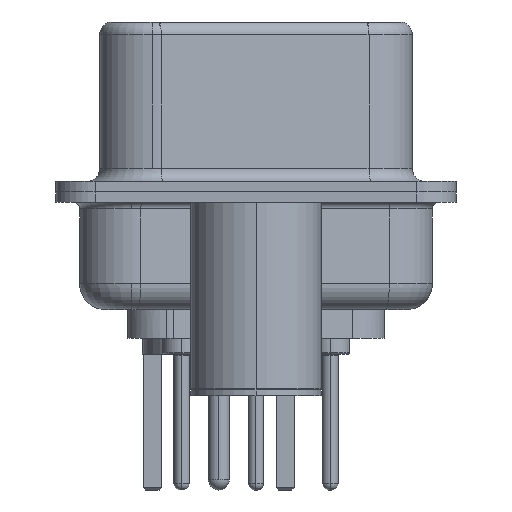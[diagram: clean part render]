
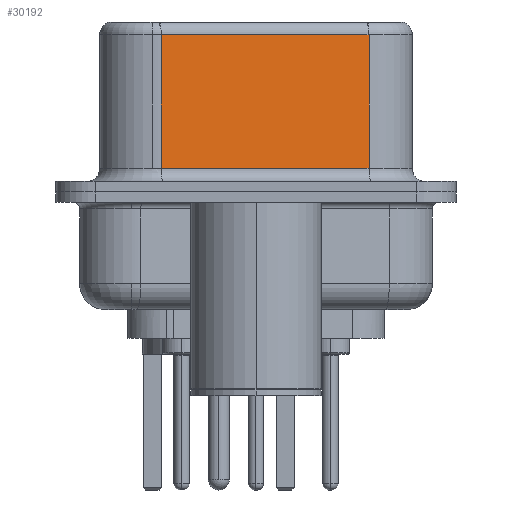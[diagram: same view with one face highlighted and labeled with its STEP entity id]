
A CAD part, left-side view. The second image highlights one B-rep face of the part: STEP entity #30192.
In plain terms, the highlighted planar face has unit normal (-0.985, -0.174, 0).
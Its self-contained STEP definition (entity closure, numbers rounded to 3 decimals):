
#232 = ORIENTED_EDGE ( 'NONE', *, *, #10060, .T. ) ;
#442 = CARTESIAN_POINT ( 'NONE',  ( 3.73, 3.628, 6.52 ) ) ;
#1006 = DIRECTION ( 'NONE',  ( 0., 0., -1. ) ) ;
#1136 = EDGE_CURVE ( 'NONE', #17221, #1732, #16563, .T. ) ;
#1732 = VERTEX_POINT ( 'NONE', #21829 ) ;
#3690 = AXIS2_PLACEMENT_3D ( 'NONE', #26724, #10558, #29506 ) ;
#3883 = VECTOR ( 'NONE', #21777, 1000. ) ;
#4448 = CARTESIAN_POINT ( 'NONE',  ( 3.73, 3.628, 0.9 ) ) ;
#5044 = PLANE ( 'NONE',  #3690 ) ;
#6447 = CARTESIAN_POINT ( 'NONE',  ( 5.132, -4.322, 0.9 ) ) ;
#8502 = VECTOR ( 'NONE', #10737, 1000. ) ;
#9507 = VECTOR ( 'NONE', #1006, 1000. ) ;
#9633 = EDGE_CURVE ( 'NONE', #17221, #12766, #16717, .T. ) ;
#10060 = EDGE_CURVE ( 'NONE', #15599, #12766, #18360, .T. ) ;
#10193 = LINE ( 'NONE', #442, #23711 ) ;
#10558 = DIRECTION ( 'NONE',  ( 0.985, 0.174, 0. ) ) ;
#10737 = DIRECTION ( 'NONE',  ( -0.174, 0.985, 0. ) ) ;
#10939 = CARTESIAN_POINT ( 'NONE',  ( 5.132, -4.322, 0.9 ) ) ;
#12766 = VERTEX_POINT ( 'NONE', #6447 ) ;
#13302 = EDGE_CURVE ( 'NONE', #1732, #15599, #10193, .T. ) ;
#13961 = DIRECTION ( 'NONE',  ( 0., 0., -1. ) ) ;
#15599 = VERTEX_POINT ( 'NONE', #4448 ) ;
#16563 = LINE ( 'NONE', #31710, #8502 ) ;
#16717 = LINE ( 'NONE', #20017, #9507 ) ;
#17221 = VERTEX_POINT ( 'NONE', #34090 ) ;
#17967 = ORIENTED_EDGE ( 'NONE', *, *, #9633, .F. ) ;
#18360 = LINE ( 'NONE', #10939, #3883 ) ;
#20017 = CARTESIAN_POINT ( 'NONE',  ( 5.132, -4.322, 6.52 ) ) ;
#21777 = DIRECTION ( 'NONE',  ( 0.174, -0.985, 0. ) ) ;
#21829 = CARTESIAN_POINT ( 'NONE',  ( 3.73, 3.628, 6.02 ) ) ;
#23711 = VECTOR ( 'NONE', #13961, 1000. ) ;
#25852 = FACE_OUTER_BOUND ( 'NONE', #28278, .T. ) ;
#26724 = CARTESIAN_POINT ( 'NONE',  ( 5.132, -4.322, 6.52 ) ) ;
#27175 = ORIENTED_EDGE ( 'NONE', *, *, #13302, .T. ) ;
#28278 = EDGE_LOOP ( 'NONE', ( #17967, #32111, #27175, #232 ) ) ;
#29506 = DIRECTION ( 'NONE',  ( -0.174, 0.985, 0. ) ) ;
#30192 = ADVANCED_FACE ( 'NONE', ( #25852 ), #5044, .F. ) ;
#31710 = CARTESIAN_POINT ( 'NONE',  ( 5.132, -4.322, 6.02 ) ) ;
#32111 = ORIENTED_EDGE ( 'NONE', *, *, #1136, .T. ) ;
#34090 = CARTESIAN_POINT ( 'NONE',  ( 5.132, -4.322, 6.02 ) ) ;
